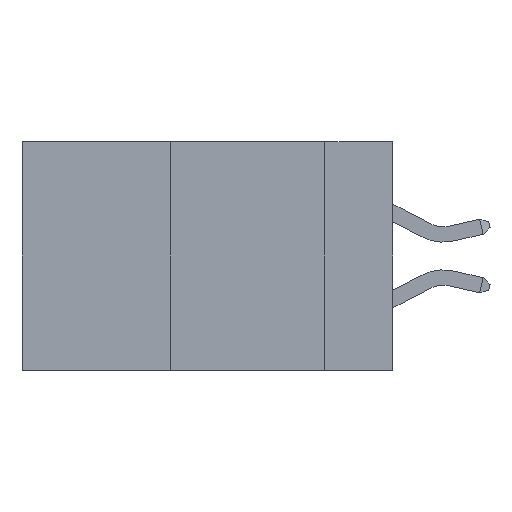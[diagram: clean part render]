
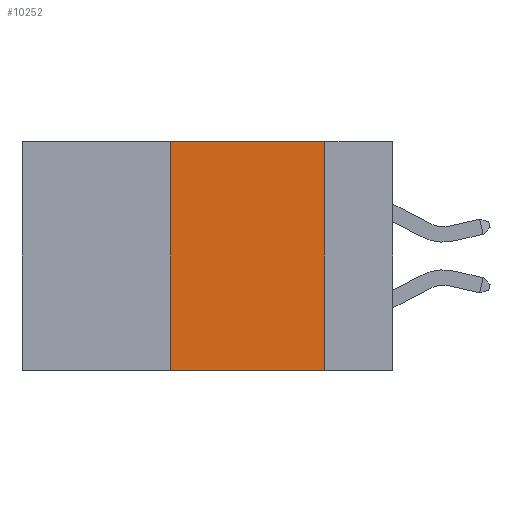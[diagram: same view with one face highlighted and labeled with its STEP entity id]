
A CAD part, left-side view. The second image highlights one B-rep face of the part: STEP entity #10252.
In plain terms, the highlighted planar face has unit normal (-1, 0, 0).
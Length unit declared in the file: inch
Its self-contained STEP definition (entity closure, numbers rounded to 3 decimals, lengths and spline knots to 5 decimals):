
#433 = CARTESIAN_POINT ( 'NONE',  ( 0., 0.6, 0. ) ) ;
#573 = AXIS2_PLACEMENT_3D ( 'NONE', #433, #4807, #14327 ) ;
#995 = EDGE_CURVE ( 'NONE', #15496, #5955, #12573, .T. ) ;
#1032 = VECTOR ( 'NONE', #9384, 39.37008 ) ;
#2682 = ORIENTED_EDGE ( 'NONE', *, *, #8531, .F. ) ;
#2752 = CARTESIAN_POINT ( 'NONE',  ( 0., 0.36, -0.37 ) ) ;
#3624 = LINE ( 'NONE', #14228, #17015 ) ;
#3870 = DIRECTION ( 'NONE',  ( 0., 0., 1. ) ) ;
#4386 = CARTESIAN_POINT ( 'NONE',  ( 0., 0.11, -0.37 ) ) ;
#4527 = DIRECTION ( 'NONE',  ( 0., 0., -1. ) ) ;
#4715 = DIRECTION ( 'NONE',  ( 0., -1., 0. ) ) ;
#4807 = DIRECTION ( 'NONE',  ( 1., 0., 0. ) ) ;
#5074 = CARTESIAN_POINT ( 'NONE',  ( 0., 0.36, 0. ) ) ;
#5396 = EDGE_CURVE ( 'NONE', #13833, #14234, #3624, .T. ) ;
#5859 = CARTESIAN_POINT ( 'NONE',  ( 0., 0.11, 0. ) ) ;
#5955 = VERTEX_POINT ( 'NONE', #4386 ) ;
#6453 = LINE ( 'NONE', #10818, #16214 ) ;
#6517 = ORIENTED_EDGE ( 'NONE', *, *, #5396, .F. ) ;
#6914 = CARTESIAN_POINT ( 'NONE',  ( 0., 0.6, -0.37 ) ) ;
#8474 = ORIENTED_EDGE ( 'NONE', *, *, #995, .T. ) ;
#8531 = EDGE_CURVE ( 'NONE', #14234, #5955, #17175, .T. ) ;
#8992 = PLANE ( 'NONE',  #573 ) ;
#9384 = DIRECTION ( 'NONE',  ( 0., -1., 0. ) ) ;
#9527 = EDGE_CURVE ( 'NONE', #15496, #13833, #6453, .T. ) ;
#10252 = ADVANCED_FACE ( 'NONE', ( #11782 ), #8992, .F. ) ;
#10376 = VECTOR ( 'NONE', #4527, 39.37008 ) ;
#10818 = CARTESIAN_POINT ( 'NONE',  ( 0., 0.36, 0. ) ) ;
#11782 = FACE_OUTER_BOUND ( 'NONE', #13633, .T. ) ;
#12573 = LINE ( 'NONE', #6914, #1032 ) ;
#13633 = EDGE_LOOP ( 'NONE', ( #2682, #6517, #15334, #8474 ) ) ;
#13833 = VERTEX_POINT ( 'NONE', #5074 ) ;
#14228 = CARTESIAN_POINT ( 'NONE',  ( 0., 0.6, 0. ) ) ;
#14234 = VERTEX_POINT ( 'NONE', #14282 ) ;
#14282 = CARTESIAN_POINT ( 'NONE',  ( 0., 0.11, 0. ) ) ;
#14327 = DIRECTION ( 'NONE',  ( 0., 0., -1. ) ) ;
#15334 = ORIENTED_EDGE ( 'NONE', *, *, #9527, .F. ) ;
#15496 = VERTEX_POINT ( 'NONE', #2752 ) ;
#16214 = VECTOR ( 'NONE', #3870, 39.37008 ) ;
#17015 = VECTOR ( 'NONE', #4715, 39.37008 ) ;
#17175 = LINE ( 'NONE', #5859, #10376 ) ;
